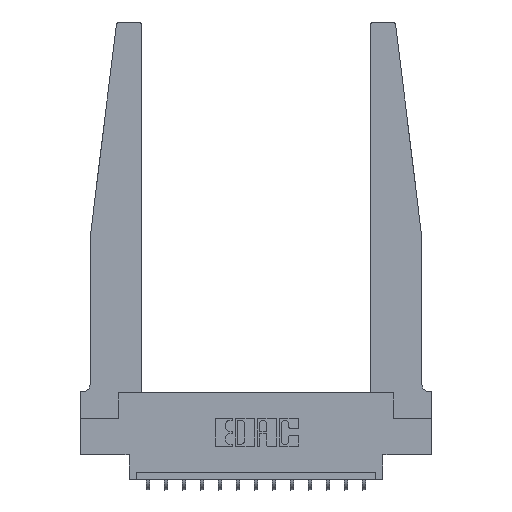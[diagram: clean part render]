
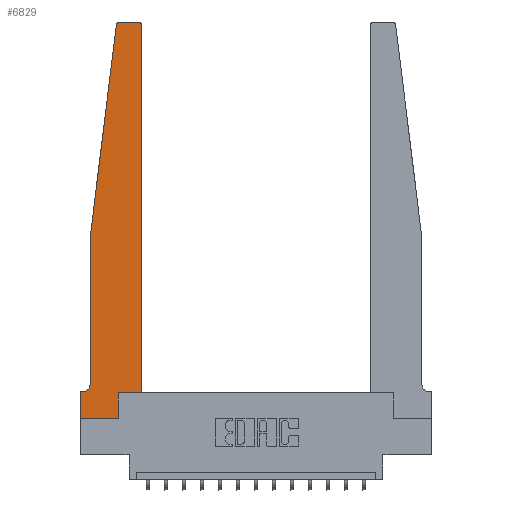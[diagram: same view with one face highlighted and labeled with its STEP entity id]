
A CAD part, top view. The second image highlights one B-rep face of the part: STEP entity #6829.
In plain terms, the highlighted planar face has unit normal (0, 0, 1).
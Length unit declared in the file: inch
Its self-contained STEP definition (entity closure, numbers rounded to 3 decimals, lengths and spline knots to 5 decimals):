
#7 = AXIS2_PLACEMENT_3D ( 'NONE', #11519, #3684, #12834 ) ;
#186 = EDGE_CURVE ( 'NONE', #16672, #7380, #10144, .T. ) ;
#213 = EDGE_CURVE ( 'NONE', #4235, #16204, #3988, .T. ) ;
#285 = ORIENTED_EDGE ( 'NONE', *, *, #1191, .T. ) ;
#478 = CARTESIAN_POINT ( 'NONE',  ( 0.395, 2.75, 0.37 ) ) ;
#533 = EDGE_CURVE ( 'NONE', #16204, #12202, #12572, .T. ) ;
#549 = DIRECTION ( 'NONE',  ( -0.122, -0.992, 0. ) ) ;
#855 = VECTOR ( 'NONE', #1975, 39.37008 ) ;
#891 = ORIENTED_EDGE ( 'NONE', *, *, #6254, .T. ) ;
#1182 = DIRECTION ( 'NONE',  ( 1., 0., 0. ) ) ;
#1191 = EDGE_CURVE ( 'NONE', #7619, #5896, #6629, .T. ) ;
#1244 = FACE_OUTER_BOUND ( 'NONE', #11755, .T. ) ;
#1274 = CARTESIAN_POINT ( 'NONE',  ( 0.2605, 0.18, 0.37 ) ) ;
#1412 = ORIENTED_EDGE ( 'NONE', *, *, #533, .T. ) ;
#1818 = DIRECTION ( 'NONE',  ( -1., 0., 0. ) ) ;
#1975 = DIRECTION ( 'NONE',  ( 0., -1., 0. ) ) ;
#2214 = CARTESIAN_POINT ( 'NONE',  ( 0.015, 0.1875, 0.37 ) ) ;
#2313 = VERTEX_POINT ( 'NONE', #13662 ) ;
#2404 = LINE ( 'NONE', #2797, #5481 ) ;
#2504 = LINE ( 'NONE', #16053, #16016 ) ;
#2707 = AXIS2_PLACEMENT_3D ( 'NONE', #8578, #9311, #1818 ) ;
#2797 = CARTESIAN_POINT ( 'NONE',  ( 0.065, 0.1875, 0.37 ) ) ;
#3265 = ORIENTED_EDGE ( 'NONE', *, *, #213, .T. ) ;
#3282 = CARTESIAN_POINT ( 'NONE',  ( 0.425, 0.18, 0.37 ) ) ;
#3641 = CARTESIAN_POINT ( 'NONE',  ( 0.27653, 2.75, 0.37 ) ) ;
#3684 = DIRECTION ( 'NONE',  ( 0., 0., 1. ) ) ;
#3988 = LINE ( 'NONE', #8728, #16686 ) ;
#4210 = VERTEX_POINT ( 'NONE', #15386 ) ;
#4235 = VERTEX_POINT ( 'NONE', #15438 ) ;
#4775 = ORIENTED_EDGE ( 'NONE', *, *, #6370, .T. ) ;
#4873 = EDGE_CURVE ( 'NONE', #7380, #4210, #14511, .T. ) ;
#5046 = AXIS2_PLACEMENT_3D ( 'NONE', #5574, #14741, #6895 ) ;
#5481 = VECTOR ( 'NONE', #9334, 39.37008 ) ;
#5493 = EDGE_CURVE ( 'NONE', #5896, #4235, #2404, .T. ) ;
#5574 = CARTESIAN_POINT ( 'NONE',  ( 0.395, 2.72, 0.37 ) ) ;
#5817 = CARTESIAN_POINT ( 'NONE',  ( 0.2605, 0.18, 0.37 ) ) ;
#5823 = CARTESIAN_POINT ( 'NONE',  ( 0., 0., 0.37 ) ) ;
#5846 = VECTOR ( 'NONE', #549, 39.37008 ) ;
#5896 = VERTEX_POINT ( 'NONE', #2214 ) ;
#6254 = EDGE_CURVE ( 'NONE', #12789, #2313, #2504, .T. ) ;
#6370 = EDGE_CURVE ( 'NONE', #13029, #7619, #7812, .T. ) ;
#6423 = ORIENTED_EDGE ( 'NONE', *, *, #11262, .T. ) ;
#6629 = CIRCLE ( 'NONE', #2707, 0.05 ) ;
#6662 = VECTOR ( 'NONE', #12408, 39.37008 ) ;
#6738 = CARTESIAN_POINT ( 'NONE',  ( 0.065, 0.2375, 0.37 ) ) ;
#6829 = ADVANCED_FACE ( 'NONE', ( #1244 ), #7716, .T. ) ;
#6895 = DIRECTION ( 'NONE',  ( 1., 0., 0. ) ) ;
#6904 = DIRECTION ( 'NONE',  ( 0., 1., 0. ) ) ;
#7380 = VERTEX_POINT ( 'NONE', #3641 ) ;
#7619 = VERTEX_POINT ( 'NONE', #6738 ) ;
#7716 = PLANE ( 'NONE',  #15943 ) ;
#7812 = LINE ( 'NONE', #13756, #855 ) ;
#7983 = DIRECTION ( 'NONE',  ( 0., -1., 0. ) ) ;
#8275 = ORIENTED_EDGE ( 'NONE', *, *, #186, .T. ) ;
#8384 = CARTESIAN_POINT ( 'NONE',  ( 0.065, 1.25, 0.37 ) ) ;
#8578 = CARTESIAN_POINT ( 'NONE',  ( 0.015, 0.2375, 0.37 ) ) ;
#8728 = CARTESIAN_POINT ( 'NONE',  ( 0., 0., 0.37 ) ) ;
#8923 = LINE ( 'NONE', #8384, #5846 ) ;
#9048 = DIRECTION ( 'NONE',  ( 0., 0., 1. ) ) ;
#9311 = DIRECTION ( 'NONE',  ( 0., 0., -1. ) ) ;
#9334 = DIRECTION ( 'NONE',  ( -1., 0., 0. ) ) ;
#9449 = CARTESIAN_POINT ( 'NONE',  ( 0.25, 2.75, 0.37 ) ) ;
#10144 = LINE ( 'NONE', #9449, #6662 ) ;
#10159 = CIRCLE ( 'NONE', #5046, 0.03 ) ;
#10750 = VECTOR ( 'NONE', #11114, 39.37008 ) ;
#10878 = ORIENTED_EDGE ( 'NONE', *, *, #11282, .T. ) ;
#11114 = DIRECTION ( 'NONE',  ( 1., 0., 0. ) ) ;
#11148 = LINE ( 'NONE', #3282, #10750 ) ;
#11262 = EDGE_CURVE ( 'NONE', #4210, #13029, #8923, .T. ) ;
#11282 = EDGE_CURVE ( 'NONE', #12202, #13164, #15071, .T. ) ;
#11519 = CARTESIAN_POINT ( 'NONE',  ( 0.27653, 2.72, 0.37 ) ) ;
#11577 = VECTOR ( 'NONE', #14986, 39.37008 ) ;
#11701 = CARTESIAN_POINT ( 'NONE',  ( 0., 0., 0.37 ) ) ;
#11755 = EDGE_LOOP ( 'NONE', ( #8275, #12925, #6423, #4775, #285, #13851, #3265, #1412, #10878, #12746, #891, #12084 ) ) ;
#11847 = EDGE_CURVE ( 'NONE', #13164, #12789, #11148, .T. ) ;
#12003 = CARTESIAN_POINT ( 'NONE',  ( 0.425, 0.18, 0.37 ) ) ;
#12079 = CARTESIAN_POINT ( 'NONE',  ( 0.2605, 0., 0.37 ) ) ;
#12084 = ORIENTED_EDGE ( 'NONE', *, *, #13258, .T. ) ;
#12202 = VERTEX_POINT ( 'NONE', #12079 ) ;
#12408 = DIRECTION ( 'NONE',  ( -1., 0., 0. ) ) ;
#12572 = LINE ( 'NONE', #11701, #12992 ) ;
#12746 = ORIENTED_EDGE ( 'NONE', *, *, #11847, .T. ) ;
#12789 = VERTEX_POINT ( 'NONE', #12003 ) ;
#12834 = DIRECTION ( 'NONE',  ( 1., 0., 0. ) ) ;
#12925 = ORIENTED_EDGE ( 'NONE', *, *, #4873, .T. ) ;
#12992 = VECTOR ( 'NONE', #14179, 39.37008 ) ;
#13029 = VERTEX_POINT ( 'NONE', #15100 ) ;
#13164 = VERTEX_POINT ( 'NONE', #1274 ) ;
#13258 = EDGE_CURVE ( 'NONE', #2313, #16672, #10159, .T. ) ;
#13662 = CARTESIAN_POINT ( 'NONE',  ( 0.425, 2.72, 0.37 ) ) ;
#13756 = CARTESIAN_POINT ( 'NONE',  ( 0.065, 1.25, 0.37 ) ) ;
#13851 = ORIENTED_EDGE ( 'NONE', *, *, #5493, .T. ) ;
#14179 = DIRECTION ( 'NONE',  ( 1., 0., 0. ) ) ;
#14511 = CIRCLE ( 'NONE', #7, 0.03 ) ;
#14741 = DIRECTION ( 'NONE',  ( 0., 0., 1. ) ) ;
#14986 = DIRECTION ( 'NONE',  ( 0., 1., 0. ) ) ;
#15071 = LINE ( 'NONE', #5817, #11577 ) ;
#15100 = CARTESIAN_POINT ( 'NONE',  ( 0.065, 1.25, 0.37 ) ) ;
#15386 = CARTESIAN_POINT ( 'NONE',  ( 0.24675, 2.72367, 0.37 ) ) ;
#15438 = CARTESIAN_POINT ( 'NONE',  ( 0., 0.1875, 0.37 ) ) ;
#15943 = AXIS2_PLACEMENT_3D ( 'NONE', #16881, #9048, #1182 ) ;
#16016 = VECTOR ( 'NONE', #6904, 39.37008 ) ;
#16053 = CARTESIAN_POINT ( 'NONE',  ( 0.425, 0.18, 0.37 ) ) ;
#16204 = VERTEX_POINT ( 'NONE', #5823 ) ;
#16672 = VERTEX_POINT ( 'NONE', #478 ) ;
#16686 = VECTOR ( 'NONE', #7983, 39.37008 ) ;
#16881 = CARTESIAN_POINT ( 'NONE',  ( 0., 0.1875, 0.37 ) ) ;
